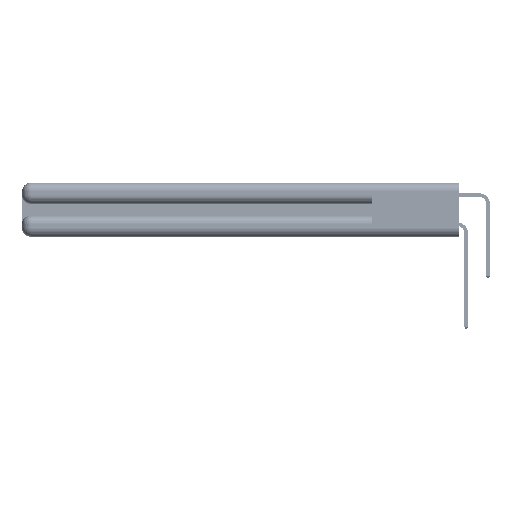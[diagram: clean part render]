
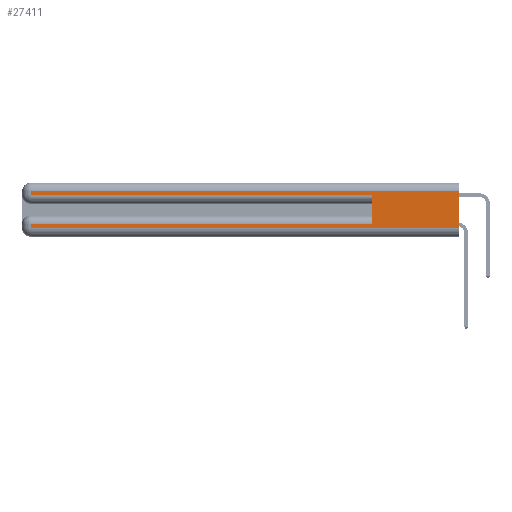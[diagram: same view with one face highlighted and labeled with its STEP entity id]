
A CAD part, left-side view. The second image highlights one B-rep face of the part: STEP entity #27411.
In plain terms, the highlighted planar face has unit normal (-1, 0, 0).
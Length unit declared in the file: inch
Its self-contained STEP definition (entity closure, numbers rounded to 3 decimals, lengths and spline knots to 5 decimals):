
#1287 = VERTEX_POINT ( 'NONE', #36003 ) ;
#1437 = EDGE_CURVE ( 'NONE', #2355, #36138, #24700, .T. ) ;
#1448 = VERTEX_POINT ( 'NONE', #20572 ) ;
#2355 = VERTEX_POINT ( 'NONE', #10822 ) ;
#2393 = VERTEX_POINT ( 'NONE', #19232 ) ;
#2825 = DIRECTION ( 'NONE',  ( 0., -1., 0. ) ) ;
#4037 = ORIENTED_EDGE ( 'NONE', *, *, #51361, .F. ) ;
#4372 = VERTEX_POINT ( 'NONE', #21596 ) ;
#5262 = LINE ( 'NONE', #47102, #15028 ) ;
#6070 = CARTESIAN_POINT ( 'NONE',  ( 0., 0., 0.37 ) ) ;
#8191 = DIRECTION ( 'NONE',  ( 0., -1., 0. ) ) ;
#8947 = VECTOR ( 'NONE', #22249, 39.37008 ) ;
#9388 = EDGE_CURVE ( 'NONE', #44225, #1287, #47183, .T. ) ;
#9570 = VECTOR ( 'NONE', #19566, 39.37008 ) ;
#9861 = CARTESIAN_POINT ( 'NONE',  ( 0., 0.6, 0.085 ) ) ;
#10054 = CARTESIAN_POINT ( 'NONE',  ( 0., 2.94, 0.37 ) ) ;
#10822 = CARTESIAN_POINT ( 'NONE',  ( 0., 2.94, 0.285 ) ) ;
#11139 = EDGE_CURVE ( 'NONE', #2393, #4372, #19860, .T. ) ;
#11373 = EDGE_CURVE ( 'NONE', #2393, #1448, #19183, .T. ) ;
#14361 = EDGE_CURVE ( 'NONE', #4372, #2355, #28415, .T. ) ;
#14602 = DIRECTION ( 'NONE',  ( 1., 0., 0. ) ) ;
#15028 = VECTOR ( 'NONE', #18862, 39.37008 ) ;
#16081 = CARTESIAN_POINT ( 'NONE',  ( 0., 2.94, 0.06 ) ) ;
#16763 = VECTOR ( 'NONE', #2825, 39.37008 ) ;
#18018 = LINE ( 'NONE', #31736, #16763 ) ;
#18862 = DIRECTION ( 'NONE',  ( 0., 0., 1. ) ) ;
#19157 = VERTEX_POINT ( 'NONE', #16081 ) ;
#19183 = LINE ( 'NONE', #35683, #9570 ) ;
#19232 = CARTESIAN_POINT ( 'NONE',  ( 0., 0., 0.31 ) ) ;
#19566 = DIRECTION ( 'NONE',  ( 0., 0., -1. ) ) ;
#19860 = LINE ( 'NONE', #38355, #8947 ) ;
#20572 = CARTESIAN_POINT ( 'NONE',  ( 0., 0., 0.06 ) ) ;
#21596 = CARTESIAN_POINT ( 'NONE',  ( 0., 2.94, 0.31 ) ) ;
#22249 = DIRECTION ( 'NONE',  ( 0., 1., 0. ) ) ;
#22438 = AXIS2_PLACEMENT_3D ( 'NONE', #6070, #14602, #42922 ) ;
#24700 = LINE ( 'NONE', #52664, #35484 ) ;
#26268 = CARTESIAN_POINT ( 'NONE',  ( 0., 0.6, 0.285 ) ) ;
#26693 = DIRECTION ( 'NONE',  ( 0., 1., 0. ) ) ;
#27091 = EDGE_LOOP ( 'NONE', ( #45084, #35997, #29172, #31889, #4037, #29654, #35627, #32249 ) ) ;
#27411 = ADVANCED_FACE ( 'NONE', ( #42016 ), #38913, .F. ) ;
#28321 = EDGE_CURVE ( 'NONE', #1287, #19157, #52603, .T. ) ;
#28415 = LINE ( 'NONE', #10054, #36627 ) ;
#29172 = ORIENTED_EDGE ( 'NONE', *, *, #14361, .T. ) ;
#29654 = ORIENTED_EDGE ( 'NONE', *, *, #9388, .T. ) ;
#30227 = DIRECTION ( 'NONE',  ( 0., 0., -1. ) ) ;
#31736 = CARTESIAN_POINT ( 'NONE',  ( 0., 0., 0.06 ) ) ;
#31889 = ORIENTED_EDGE ( 'NONE', *, *, #1437, .T. ) ;
#32249 = ORIENTED_EDGE ( 'NONE', *, *, #37114, .T. ) ;
#34455 = DIRECTION ( 'NONE',  ( 0., 0., -1. ) ) ;
#35484 = VECTOR ( 'NONE', #8191, 39.37008 ) ;
#35627 = ORIENTED_EDGE ( 'NONE', *, *, #28321, .T. ) ;
#35683 = CARTESIAN_POINT ( 'NONE',  ( 0., 0., 0.37 ) ) ;
#35997 = ORIENTED_EDGE ( 'NONE', *, *, #11139, .T. ) ;
#36003 = CARTESIAN_POINT ( 'NONE',  ( 0., 2.94, 0.085 ) ) ;
#36138 = VERTEX_POINT ( 'NONE', #26268 ) ;
#36530 = VECTOR ( 'NONE', #26693, 39.37008 ) ;
#36627 = VECTOR ( 'NONE', #34455, 39.37008 ) ;
#37114 = EDGE_CURVE ( 'NONE', #19157, #1448, #18018, .T. ) ;
#38163 = CARTESIAN_POINT ( 'NONE',  ( 0., 2.94, 0.37 ) ) ;
#38355 = CARTESIAN_POINT ( 'NONE',  ( 0., 0., 0.31 ) ) ;
#38711 = CARTESIAN_POINT ( 'NONE',  ( 0., 0., 0.085 ) ) ;
#38913 = PLANE ( 'NONE',  #22438 ) ;
#42016 = FACE_OUTER_BOUND ( 'NONE', #27091, .T. ) ;
#42922 = DIRECTION ( 'NONE',  ( 0., 0., -1. ) ) ;
#44225 = VERTEX_POINT ( 'NONE', #9861 ) ;
#45084 = ORIENTED_EDGE ( 'NONE', *, *, #11373, .F. ) ;
#47102 = CARTESIAN_POINT ( 'NONE',  ( 0., 0.6, 0.145 ) ) ;
#47183 = LINE ( 'NONE', #38711, #36530 ) ;
#51341 = VECTOR ( 'NONE', #30227, 39.37008 ) ;
#51361 = EDGE_CURVE ( 'NONE', #44225, #36138, #5262, .T. ) ;
#52603 = LINE ( 'NONE', #38163, #51341 ) ;
#52664 = CARTESIAN_POINT ( 'NONE',  ( 0., 0., 0.285 ) ) ;
